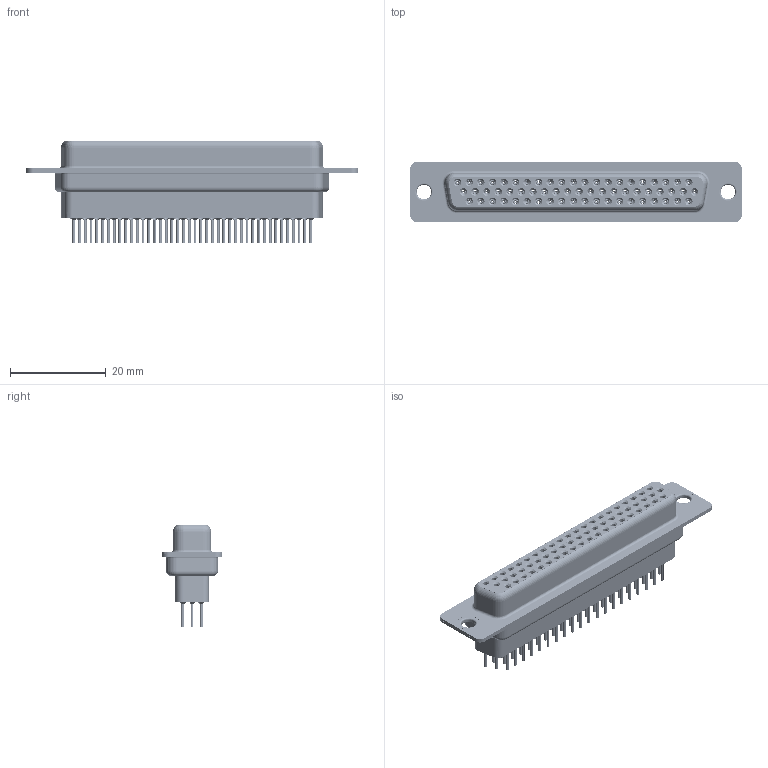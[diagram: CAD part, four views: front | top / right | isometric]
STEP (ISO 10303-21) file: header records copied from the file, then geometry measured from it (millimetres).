
FILE_DESCRIPTION (( 'STEP AP203' ), '1' );
FILE_NAME ('638-062-631-051.STEP', '2020-07-19T02:47:31', ( '' ), ( '' ), 'SwSTEP 2.0', 'SolidWorks 2020', '' );
FILE_SCHEMA (( 'CONFIG_CONTROL_DESIGN' ));
Length unit declared in the file: millimetre
Products named in the file (8): 638 Contact Row 3_31; 638-062-631-051; 638 Shell Rear_62 Contacts; 638 Housing_62 Contacts HP; 638 Shell Front_62 Contacts; 638 Contact Row 2_31; 638 Thru Hole Rivet; 638 Contact Row 1_31
Assembly tree (67 placements, depth 2):
  638-062-631-051
    638 Housing_62 Contacts HP
    638 Shell Front_62 Contacts
    638 Shell Rear_62 Contacts
    638 Contact Row 1_31  x21
    638 Contact Row 2_31  x21
    638 Contact Row 3_31  x20
    638 Thru Hole Rivet  x2
Bounding box: 69.32 x 12.6 x 21.5 mm (x, y, z)
Volume: 5564.1 mm3; surface area: 20971.6 mm2
Topology: 67 solids, 67 shells, 7879 faces, 20195 edges, 12585 vertices
Faces by surface type: cylinder 2167, plane 1989, torus 1553, bspline 1240, cone 930
Entity records: 45063 total; most frequent: CARTESIAN_POINT 10332, DIRECTION 7293, ORIENTED_EDGE 6320, EDGE_CURVE 3160, AXIS2_PLACEMENT_3D 3090, VERTEX_POINT 2000, CIRCLE 1711, EDGE_LOOP 1702
